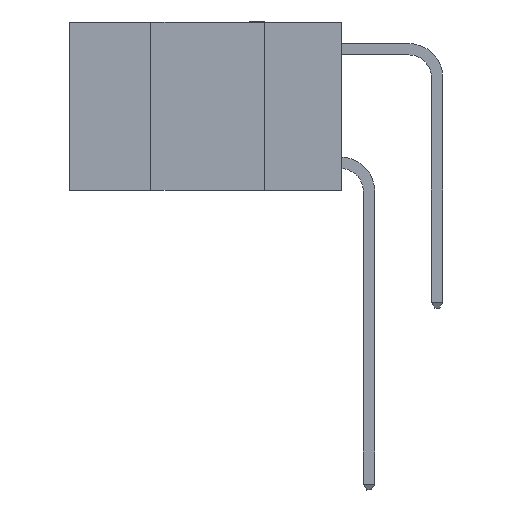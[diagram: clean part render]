
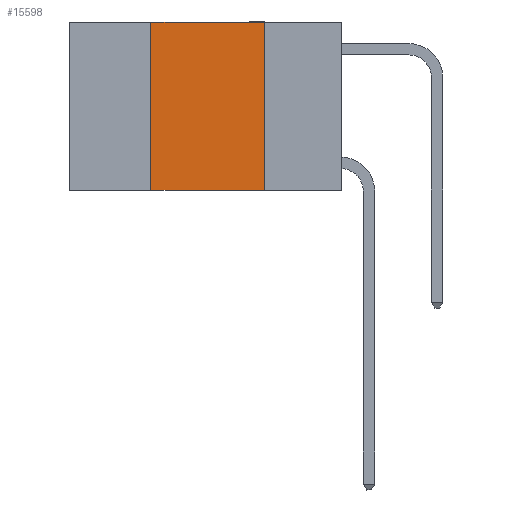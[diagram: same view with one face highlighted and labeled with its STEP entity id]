
A CAD part, left-side view. The second image highlights one B-rep face of the part: STEP entity #15598.
In plain terms, the highlighted planar face has unit normal (-1, 0, 0).
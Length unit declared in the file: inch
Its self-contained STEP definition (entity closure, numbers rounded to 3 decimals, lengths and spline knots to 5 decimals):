
#223 = EDGE_LOOP ( 'NONE', ( #13559, #1857, #10480, #17476 ) ) ;
#329 = DIRECTION ( 'NONE',  ( 0., 0., -1. ) ) ;
#1857 = ORIENTED_EDGE ( 'NONE', *, *, #18588, .F. ) ;
#2515 = VECTOR ( 'NONE', #18494, 39.37008 ) ;
#2676 = AXIS2_PLACEMENT_3D ( 'NONE', #18741, #3213, #329 ) ;
#3213 = DIRECTION ( 'NONE',  ( 1., 0., 0. ) ) ;
#3778 = EDGE_CURVE ( 'NONE', #16351, #20096, #10941, .T. ) ;
#3980 = CARTESIAN_POINT ( 'NONE',  ( 0., 0.17, -0.37 ) ) ;
#4936 = DIRECTION ( 'NONE',  ( 0., 0., 1. ) ) ;
#4992 = VECTOR ( 'NONE', #4936, 39.37008 ) ;
#5815 = CARTESIAN_POINT ( 'NONE',  ( 0., 0.6, -0.37 ) ) ;
#5914 = DIRECTION ( 'NONE',  ( 0., -1., 0. ) ) ;
#6343 = VECTOR ( 'NONE', #5914, 39.37008 ) ;
#6475 = LINE ( 'NONE', #12707, #4992 ) ;
#8544 = LINE ( 'NONE', #12117, #17401 ) ;
#10111 = LINE ( 'NONE', #5815, #6343 ) ;
#10480 = ORIENTED_EDGE ( 'NONE', *, *, #12786, .F. ) ;
#10941 = LINE ( 'NONE', #13794, #2515 ) ;
#10981 = FACE_OUTER_BOUND ( 'NONE', #223, .T. ) ;
#11084 = PLANE ( 'NONE',  #2676 ) ;
#11240 = CARTESIAN_POINT ( 'NONE',  ( 0., 0.42, 0. ) ) ;
#11402 = VERTEX_POINT ( 'NONE', #17395 ) ;
#12117 = CARTESIAN_POINT ( 'NONE',  ( 0., 0.6, 0. ) ) ;
#12707 = CARTESIAN_POINT ( 'NONE',  ( 0., 0.42, 0. ) ) ;
#12786 = EDGE_CURVE ( 'NONE', #11402, #18086, #6475, .T. ) ;
#13383 = CARTESIAN_POINT ( 'NONE',  ( 0., 0.17, 0. ) ) ;
#13559 = ORIENTED_EDGE ( 'NONE', *, *, #3778, .F. ) ;
#13794 = CARTESIAN_POINT ( 'NONE',  ( 0., 0.17, 0. ) ) ;
#14983 = DIRECTION ( 'NONE',  ( 0., -1., 0. ) ) ;
#15598 = ADVANCED_FACE ( 'NONE', ( #10981 ), #11084, .F. ) ;
#16351 = VERTEX_POINT ( 'NONE', #13383 ) ;
#17395 = CARTESIAN_POINT ( 'NONE',  ( 0., 0.42, -0.37 ) ) ;
#17401 = VECTOR ( 'NONE', #14983, 39.37008 ) ;
#17476 = ORIENTED_EDGE ( 'NONE', *, *, #19278, .T. ) ;
#18086 = VERTEX_POINT ( 'NONE', #11240 ) ;
#18494 = DIRECTION ( 'NONE',  ( 0., 0., -1. ) ) ;
#18588 = EDGE_CURVE ( 'NONE', #18086, #16351, #8544, .T. ) ;
#18741 = CARTESIAN_POINT ( 'NONE',  ( 0., 0.6, 0. ) ) ;
#19278 = EDGE_CURVE ( 'NONE', #11402, #20096, #10111, .T. ) ;
#20096 = VERTEX_POINT ( 'NONE', #3980 ) ;
